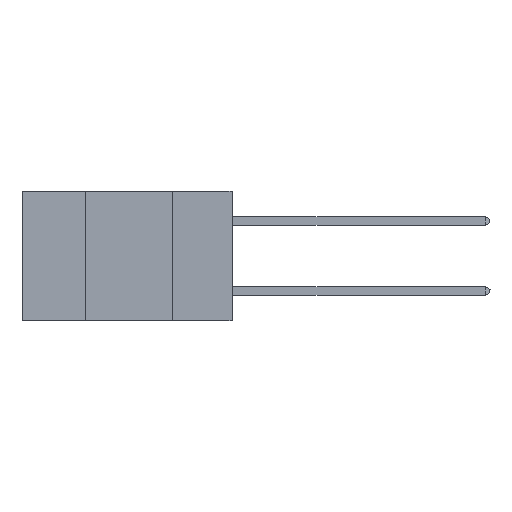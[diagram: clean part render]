
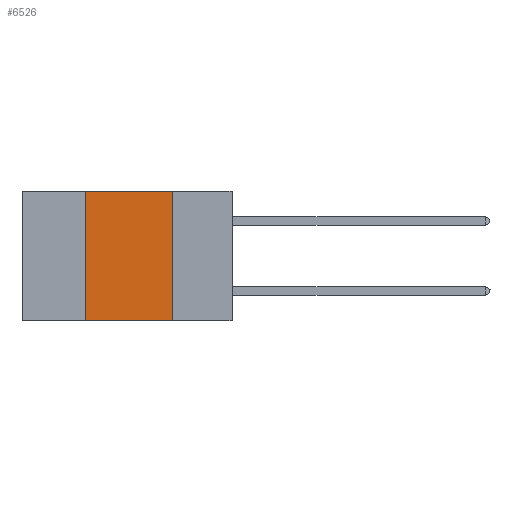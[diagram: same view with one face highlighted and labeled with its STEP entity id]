
A CAD part, left-side view. The second image highlights one B-rep face of the part: STEP entity #6526.
In plain terms, the highlighted planar face has unit normal (-1, 0, 0).
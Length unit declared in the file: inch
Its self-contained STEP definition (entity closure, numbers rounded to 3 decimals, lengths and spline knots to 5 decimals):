
#1637 = VECTOR ( 'NONE', #11491, 39.37008 ) ;
#1738 = EDGE_CURVE ( 'NONE', #10130, #19208, #16857, .T. ) ;
#3875 = EDGE_CURVE ( 'NONE', #19208, #15690, #9249, .T. ) ;
#4369 = LINE ( 'NONE', #15913, #22513 ) ;
#5948 = CARTESIAN_POINT ( 'NONE',  ( 0., 0.6, 0. ) ) ;
#6200 = VECTOR ( 'NONE', #8254, 39.37008 ) ;
#6526 = ADVANCED_FACE ( 'NONE', ( #18561 ), #14853, .F. ) ;
#6631 = VECTOR ( 'NONE', #11240, 39.37008 ) ;
#6812 = DIRECTION ( 'NONE',  ( 0., -1., 0. ) ) ;
#7827 = CARTESIAN_POINT ( 'NONE',  ( 0., 0.42, 0. ) ) ;
#7834 = ORIENTED_EDGE ( 'NONE', *, *, #9716, .T. ) ;
#8029 = ORIENTED_EDGE ( 'NONE', *, *, #1738, .F. ) ;
#8254 = DIRECTION ( 'NONE',  ( 0., 0., -1. ) ) ;
#8439 = CARTESIAN_POINT ( 'NONE',  ( 0., 0.17, -0.37 ) ) ;
#9249 = LINE ( 'NONE', #5948, #1637 ) ;
#9518 = DIRECTION ( 'NONE',  ( 0., 0., -1. ) ) ;
#9675 = VERTEX_POINT ( 'NONE', #8439 ) ;
#9716 = EDGE_CURVE ( 'NONE', #10130, #9675, #4369, .T. ) ;
#9862 = ORIENTED_EDGE ( 'NONE', *, *, #16625, .F. ) ;
#10130 = VERTEX_POINT ( 'NONE', #12216 ) ;
#11240 = DIRECTION ( 'NONE',  ( 0., 0., 1. ) ) ;
#11491 = DIRECTION ( 'NONE',  ( 0., -1., 0. ) ) ;
#12216 = CARTESIAN_POINT ( 'NONE',  ( 0., 0.42, -0.37 ) ) ;
#12962 = ORIENTED_EDGE ( 'NONE', *, *, #3875, .F. ) ;
#14771 = DIRECTION ( 'NONE',  ( 1., 0., 0. ) ) ;
#14853 = PLANE ( 'NONE',  #16070 ) ;
#15094 = CARTESIAN_POINT ( 'NONE',  ( 0., 0.42, 0. ) ) ;
#15690 = VERTEX_POINT ( 'NONE', #17460 ) ;
#15913 = CARTESIAN_POINT ( 'NONE',  ( 0., 0.6, -0.37 ) ) ;
#16070 = AXIS2_PLACEMENT_3D ( 'NONE', #18180, #14771, #9518 ) ;
#16625 = EDGE_CURVE ( 'NONE', #15690, #9675, #21049, .T. ) ;
#16719 = EDGE_LOOP ( 'NONE', ( #9862, #12962, #8029, #7834 ) ) ;
#16857 = LINE ( 'NONE', #7827, #6631 ) ;
#17068 = CARTESIAN_POINT ( 'NONE',  ( 0., 0.17, 0. ) ) ;
#17460 = CARTESIAN_POINT ( 'NONE',  ( 0., 0.17, 0. ) ) ;
#18180 = CARTESIAN_POINT ( 'NONE',  ( 0., 0.6, 0. ) ) ;
#18561 = FACE_OUTER_BOUND ( 'NONE', #16719, .T. ) ;
#19208 = VERTEX_POINT ( 'NONE', #15094 ) ;
#21049 = LINE ( 'NONE', #17068, #6200 ) ;
#22513 = VECTOR ( 'NONE', #6812, 39.37008 ) ;
